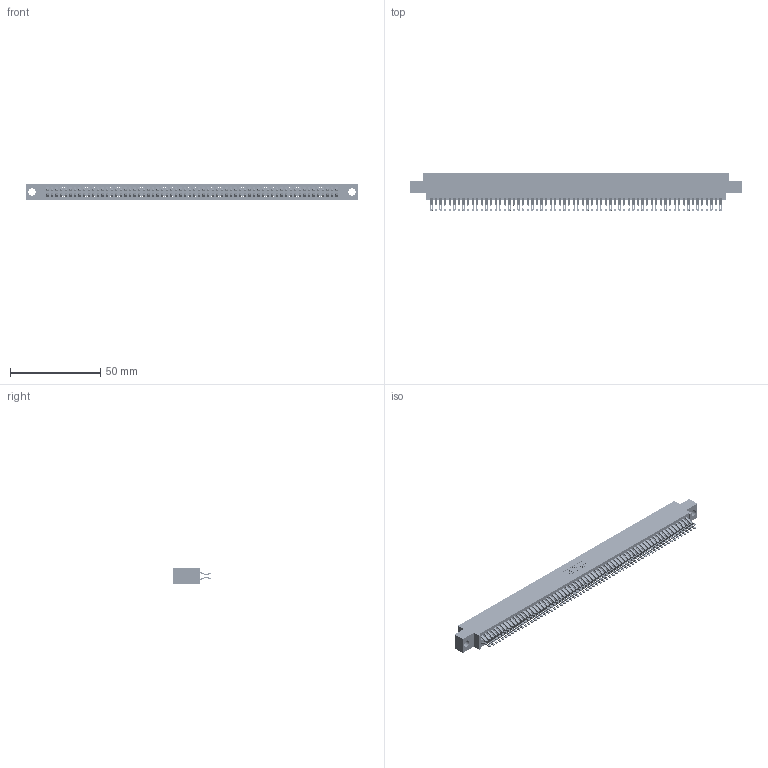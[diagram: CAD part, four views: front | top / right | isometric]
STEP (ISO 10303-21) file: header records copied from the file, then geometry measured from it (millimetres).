
FILE_DESCRIPTION (( 'STEP AP203' ), '1' );
FILE_NAME ('395-128-555-804.STEP', '2021-06-17T23:48:14', ( '' ), ( '' ), 'SwSTEP 2.0', 'SolidWorks 2020', '' );
FILE_SCHEMA (( 'CONFIG_CONTROL_DESIGN' ));
Length unit declared in the file: inch
Products named in the file (3): 345 Part_0.170 Offset - 0.156 Dia-TI; 345-292-001_555 Tail; 395-128-555-804
Assembly tree (129 placements, depth 2):
  395-128-555-804
    345 Part_0.170 Offset - 0.156 Dia-TI
    345-292-001_555 Tail  x128
Bounding box: 183.77 x 21.13 x 9.4 mm (x, y, z)
Volume: 18207.7 mm3; surface area: 28626.4 mm2
Topology: 129 solids, 129 shells, 7312 faces, 23045 edges, 15362 vertices
Faces by surface type: plane 4066, cylinder 3246
Entity records: 48131 total; most frequent: CARTESIAN_POINT 8088, ORIENTED_EDGE 7990, DIRECTION 7071, EDGE_CURVE 3995, LINE 3587, VECTOR 3587, VERTEX_POINT 2662, AXIS2_PLACEMENT_3D 1742
